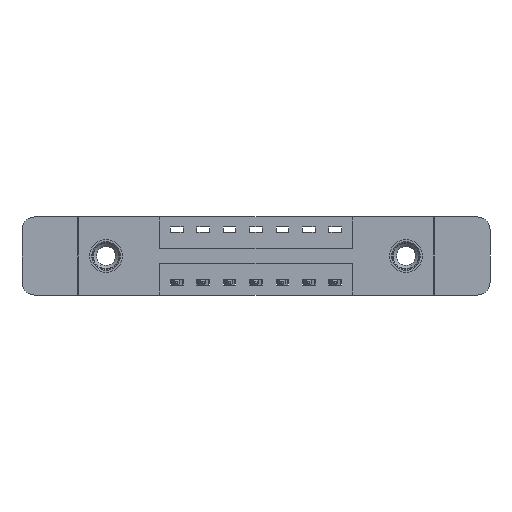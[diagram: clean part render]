
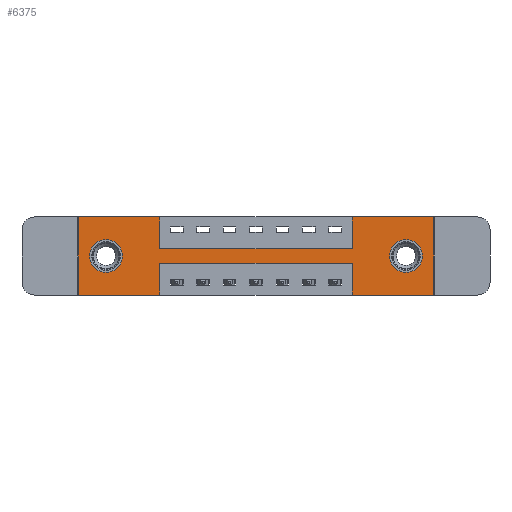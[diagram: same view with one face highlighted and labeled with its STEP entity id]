
A CAD part, front view. The second image highlights one B-rep face of the part: STEP entity #6375.
In plain terms, the highlighted planar face has unit normal (0, -1, 0).
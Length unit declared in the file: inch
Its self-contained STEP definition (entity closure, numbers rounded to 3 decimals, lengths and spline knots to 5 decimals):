
#10 = ORIENTED_EDGE ( 'NONE', *, *, #13215, .F. ) ;
#60 = VERTEX_POINT ( 'NONE', #14399 ) ;
#108 = VERTEX_POINT ( 'NONE', #923 ) ;
#309 = DIRECTION ( 'NONE',  ( 0., 0., -1. ) ) ;
#410 = VECTOR ( 'NONE', #2414, 39.37008 ) ;
#423 = DIRECTION ( 'NONE',  ( 0., 1., 0. ) ) ;
#694 = EDGE_CURVE ( 'NONE', #60, #5174, #8616, .T. ) ;
#827 = VERTEX_POINT ( 'NONE', #4033 ) ;
#923 = CARTESIAN_POINT ( 'NONE',  ( 0.1325, 0., -0.263 ) ) ;
#927 = DIRECTION ( 'NONE',  ( -1., 0., 0. ) ) ;
#1069 = ORIENTED_EDGE ( 'NONE', *, *, #10271, .F. ) ;
#1103 = ORIENTED_EDGE ( 'NONE', *, *, #1993, .F. ) ;
#1185 = CARTESIAN_POINT ( 'NONE',  ( 0., 0., -0.37 ) ) ;
#1228 = VERTEX_POINT ( 'NONE', #6733 ) ;
#1240 = CARTESIAN_POINT ( 'NONE',  ( 0., 0., -0.37 ) ) ;
#1259 = DIRECTION ( 'NONE',  ( 0., -1., 0. ) ) ;
#1298 = LINE ( 'NONE', #10303, #12987 ) ;
#1514 = LINE ( 'NONE', #10304, #410 ) ;
#1528 = EDGE_LOOP ( 'NONE', ( #6590, #13982 ) ) ;
#1629 = LINE ( 'NONE', #5875, #12015 ) ;
#1634 = DIRECTION ( 'NONE',  ( 0., 0., 1. ) ) ;
#1846 = DIRECTION ( 'NONE',  ( -1., 0., 0. ) ) ;
#1853 = VERTEX_POINT ( 'NONE', #11372 ) ;
#1993 = EDGE_CURVE ( 'NONE', #7757, #1853, #11581, .T. ) ;
#2156 = ORIENTED_EDGE ( 'NONE', *, *, #8296, .F. ) ;
#2176 = DIRECTION ( 'NONE',  ( 0., 0., -1. ) ) ;
#2211 = CIRCLE ( 'NONE', #14313, 0.078 ) ;
#2309 = VERTEX_POINT ( 'NONE', #10171 ) ;
#2318 = LINE ( 'NONE', #11359, #8278 ) ;
#2414 = DIRECTION ( 'NONE',  ( 1., 0., 0. ) ) ;
#2449 = FACE_BOUND ( 'NONE', #9524, .T. ) ;
#2544 = CARTESIAN_POINT ( 'NONE',  ( 1.685, 0., 0. ) ) ;
#2661 = CARTESIAN_POINT ( 'NONE',  ( 1.5525, 0., -0.107 ) ) ;
#2743 = VERTEX_POINT ( 'NONE', #8502 ) ;
#2750 = CIRCLE ( 'NONE', #14626, 0.078 ) ;
#2754 = EDGE_CURVE ( 'NONE', #2309, #1228, #6496, .T. ) ;
#2842 = LINE ( 'NONE', #9588, #11741 ) ;
#2903 = VECTOR ( 'NONE', #7707, 39.37008 ) ;
#3139 = CARTESIAN_POINT ( 'NONE',  ( 0.3875, 0., -0.22 ) ) ;
#3361 = ORIENTED_EDGE ( 'NONE', *, *, #4416, .F. ) ;
#3545 = DIRECTION ( 'NONE',  ( 0., 0., -1. ) ) ;
#3550 = DIRECTION ( 'NONE',  ( 0., 0., -1. ) ) ;
#3706 = DIRECTION ( 'NONE',  ( 0., 0., 1. ) ) ;
#3761 = EDGE_CURVE ( 'NONE', #11845, #4255, #6550, .T. ) ;
#3886 = ORIENTED_EDGE ( 'NONE', *, *, #3761, .F. ) ;
#4033 = CARTESIAN_POINT ( 'NONE',  ( 1.2975, 0., 0. ) ) ;
#4255 = VERTEX_POINT ( 'NONE', #1240 ) ;
#4375 = VECTOR ( 'NONE', #3550, 39.37008 ) ;
#4416 = EDGE_CURVE ( 'NONE', #827, #7757, #1629, .T. ) ;
#4539 = FACE_BOUND ( 'NONE', #1528, .T. ) ;
#4872 = DIRECTION ( 'NONE',  ( 0., 0., -1. ) ) ;
#4906 = CIRCLE ( 'NONE', #7281, 0.078 ) ;
#5149 = VERTEX_POINT ( 'NONE', #9238 ) ;
#5174 = VERTEX_POINT ( 'NONE', #12769 ) ;
#5224 = EDGE_CURVE ( 'NONE', #10522, #2743, #4906, .T. ) ;
#5276 = VERTEX_POINT ( 'NONE', #14258 ) ;
#5587 = ORIENTED_EDGE ( 'NONE', *, *, #5224, .T. ) ;
#5594 = VECTOR ( 'NONE', #11997, 39.37008 ) ;
#5750 = EDGE_CURVE ( 'NONE', #108, #5276, #2750, .T. ) ;
#5825 = DIRECTION ( 'NONE',  ( 1., 0., 0. ) ) ;
#5875 = CARTESIAN_POINT ( 'NONE',  ( 0., 0., 0. ) ) ;
#5878 = DIRECTION ( 'NONE',  ( 0., 1., 0. ) ) ;
#5940 = EDGE_LOOP ( 'NONE', ( #2156, #1069, #7816, #7999, #1103, #3361, #13381, #8132, #13120, #7489, #10, #3886 ) ) ;
#6004 = CIRCLE ( 'NONE', #9327, 0.078 ) ;
#6069 = VECTOR ( 'NONE', #14365, 39.37008 ) ;
#6284 = LINE ( 'NONE', #10851, #12710 ) ;
#6321 = CARTESIAN_POINT ( 'NONE',  ( 0., 0., -0.37 ) ) ;
#6355 = EDGE_CURVE ( 'NONE', #1228, #11240, #1514, .T. ) ;
#6375 = ADVANCED_FACE ( 'NONE', ( #2449, #4539, #8031 ), #7080, .T. ) ;
#6496 = LINE ( 'NONE', #12318, #6069 ) ;
#6550 = LINE ( 'NONE', #6321, #8634 ) ;
#6590 = ORIENTED_EDGE ( 'NONE', *, *, #7412, .T. ) ;
#6733 = CARTESIAN_POINT ( 'NONE',  ( 0.3875, 0., -0.15 ) ) ;
#6813 = EDGE_CURVE ( 'NONE', #5149, #2309, #2318, .T. ) ;
#6968 = VERTEX_POINT ( 'NONE', #10218 ) ;
#7080 = PLANE ( 'NONE',  #13008 ) ;
#7281 = AXIS2_PLACEMENT_3D ( 'NONE', #13993, #9460, #309 ) ;
#7343 = DIRECTION ( 'NONE',  ( 0., 0., 1. ) ) ;
#7412 = EDGE_CURVE ( 'NONE', #5276, #108, #2211, .T. ) ;
#7489 = ORIENTED_EDGE ( 'NONE', *, *, #6813, .F. ) ;
#7707 = DIRECTION ( 'NONE',  ( -1., 0., 0. ) ) ;
#7757 = VERTEX_POINT ( 'NONE', #2544 ) ;
#7781 = LINE ( 'NONE', #3139, #14060 ) ;
#7816 = ORIENTED_EDGE ( 'NONE', *, *, #694, .F. ) ;
#7885 = EDGE_CURVE ( 'NONE', #2743, #10522, #6004, .T. ) ;
#7999 = ORIENTED_EDGE ( 'NONE', *, *, #8652, .F. ) ;
#8031 = FACE_OUTER_BOUND ( 'NONE', #5940, .T. ) ;
#8064 = DIRECTION ( 'NONE',  ( 0., 0., 1. ) ) ;
#8132 = ORIENTED_EDGE ( 'NONE', *, *, #6355, .F. ) ;
#8278 = VECTOR ( 'NONE', #5825, 39.37008 ) ;
#8296 = EDGE_CURVE ( 'NONE', #6968, #11845, #6284, .T. ) ;
#8502 = CARTESIAN_POINT ( 'NONE',  ( 1.5525, 0., -0.263 ) ) ;
#8616 = LINE ( 'NONE', #13106, #5594 ) ;
#8634 = VECTOR ( 'NONE', #1846, 39.37008 ) ;
#8652 = EDGE_CURVE ( 'NONE', #1853, #60, #14481, .T. ) ;
#8831 = CARTESIAN_POINT ( 'NONE',  ( 0., 0., -0.37 ) ) ;
#9238 = CARTESIAN_POINT ( 'NONE',  ( 0., 0., 0. ) ) ;
#9265 = CARTESIAN_POINT ( 'NONE',  ( 1.2975, 0., -0.15 ) ) ;
#9294 = CARTESIAN_POINT ( 'NONE',  ( 0.1325, 0., -0.185 ) ) ;
#9322 = CARTESIAN_POINT ( 'NONE',  ( 1.5525, 0., -0.185 ) ) ;
#9327 = AXIS2_PLACEMENT_3D ( 'NONE', #9322, #423, #4872 ) ;
#9460 = DIRECTION ( 'NONE',  ( 0., 1., 0. ) ) ;
#9524 = EDGE_LOOP ( 'NONE', ( #5587, #9671 ) ) ;
#9588 = CARTESIAN_POINT ( 'NONE',  ( 1.2975, 0., 0. ) ) ;
#9671 = ORIENTED_EDGE ( 'NONE', *, *, #7885, .T. ) ;
#10139 = EDGE_CURVE ( 'NONE', #11240, #827, #2842, .T. ) ;
#10171 = CARTESIAN_POINT ( 'NONE',  ( 0.3875, 0., 0. ) ) ;
#10218 = CARTESIAN_POINT ( 'NONE',  ( 0.3875, 0., -0.22 ) ) ;
#10271 = EDGE_CURVE ( 'NONE', #5174, #6968, #7781, .T. ) ;
#10303 = CARTESIAN_POINT ( 'NONE',  ( 0., 0., 0. ) ) ;
#10304 = CARTESIAN_POINT ( 'NONE',  ( 0.3875, 0., -0.15 ) ) ;
#10522 = VERTEX_POINT ( 'NONE', #2661 ) ;
#10651 = DIRECTION ( 'NONE',  ( 0., 1., 0. ) ) ;
#10851 = CARTESIAN_POINT ( 'NONE',  ( 0.3875, 0., -0.37 ) ) ;
#11240 = VERTEX_POINT ( 'NONE', #9265 ) ;
#11359 = CARTESIAN_POINT ( 'NONE',  ( 0., 0., 0. ) ) ;
#11372 = CARTESIAN_POINT ( 'NONE',  ( 1.685, 0., -0.37 ) ) ;
#11581 = LINE ( 'NONE', #12902, #4375 ) ;
#11741 = VECTOR ( 'NONE', #1634, 39.37008 ) ;
#11845 = VERTEX_POINT ( 'NONE', #13520 ) ;
#11997 = DIRECTION ( 'NONE',  ( 0., 0., 1. ) ) ;
#12015 = VECTOR ( 'NONE', #12743, 39.37008 ) ;
#12318 = CARTESIAN_POINT ( 'NONE',  ( 0.3875, 0., 0. ) ) ;
#12710 = VECTOR ( 'NONE', #2176, 39.37008 ) ;
#12743 = DIRECTION ( 'NONE',  ( 1., 0., 0. ) ) ;
#12769 = CARTESIAN_POINT ( 'NONE',  ( 1.2975, 0., -0.22 ) ) ;
#12902 = CARTESIAN_POINT ( 'NONE',  ( 1.685, 0., 0. ) ) ;
#12987 = VECTOR ( 'NONE', #8064, 39.37008 ) ;
#13008 = AXIS2_PLACEMENT_3D ( 'NONE', #1185, #1259, #3545 ) ;
#13106 = CARTESIAN_POINT ( 'NONE',  ( 1.2975, 0., -0.37 ) ) ;
#13120 = ORIENTED_EDGE ( 'NONE', *, *, #2754, .F. ) ;
#13215 = EDGE_CURVE ( 'NONE', #4255, #5149, #1298, .T. ) ;
#13381 = ORIENTED_EDGE ( 'NONE', *, *, #10139, .F. ) ;
#13520 = CARTESIAN_POINT ( 'NONE',  ( 0.3875, 0., -0.37 ) ) ;
#13973 = CARTESIAN_POINT ( 'NONE',  ( 0.1325, 0., -0.185 ) ) ;
#13982 = ORIENTED_EDGE ( 'NONE', *, *, #5750, .T. ) ;
#13993 = CARTESIAN_POINT ( 'NONE',  ( 1.5525, 0., -0.185 ) ) ;
#14060 = VECTOR ( 'NONE', #927, 39.37008 ) ;
#14258 = CARTESIAN_POINT ( 'NONE',  ( 0.1325, 0., -0.107 ) ) ;
#14313 = AXIS2_PLACEMENT_3D ( 'NONE', #13973, #10651, #7343 ) ;
#14365 = DIRECTION ( 'NONE',  ( 0., 0., -1. ) ) ;
#14399 = CARTESIAN_POINT ( 'NONE',  ( 1.2975, 0., -0.37 ) ) ;
#14481 = LINE ( 'NONE', #8831, #2903 ) ;
#14626 = AXIS2_PLACEMENT_3D ( 'NONE', #9294, #5878, #3706 ) ;
